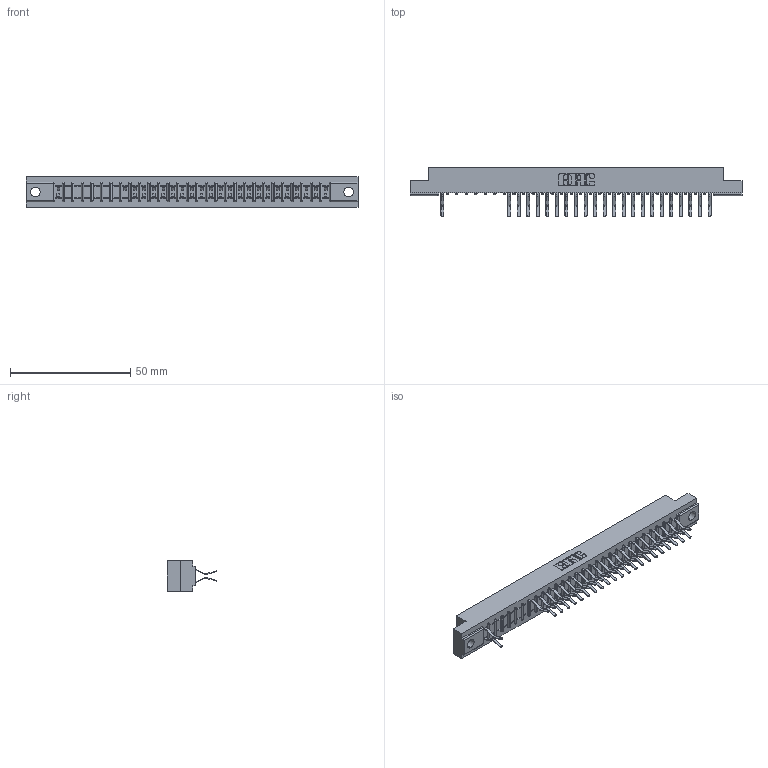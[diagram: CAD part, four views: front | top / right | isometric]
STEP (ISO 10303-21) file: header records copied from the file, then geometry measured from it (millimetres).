
FILE_DESCRIPTION (( 'STEP AP203' ), '1' );
FILE_NAME ('307-058-560-202.STEP', '2018-08-06T08:02:11', ( '' ), ( '' ), 'SwSTEP 2.0', 'SolidWorks 2016', '' );
FILE_SCHEMA (( 'CONFIG_CONTROL_DESIGN' ));
Length unit declared in the file: inch
Products named in the file (3): 307 Part_.128 Dia Mounting Holes; 307-290-001_560; 307-058-560-202
Assembly tree (46 placements, depth 2):
  307-058-560-202
    307 Part_.128 Dia Mounting Holes
    307-290-001_560  x45
Bounding box: 137.92 x 20.73 x 12.7 mm (x, y, z)
Volume: 14374.2 mm3; surface area: 16323.6 mm2
Topology: 46 solids, 46 shells, 2528 faces, 7129 edges, 4610 vertices
Faces by surface type: plane 1633, cylinder 835, sphere 60
Entity records: 27082 total; most frequent: CARTESIAN_POINT 4488, ORIENTED_EDGE 4458, DIRECTION 4389, EDGE_CURVE 2229, VECTOR 1703, LINE 1703, VERTEX_POINT 1442, AXIS2_PLACEMENT_3D 1343
